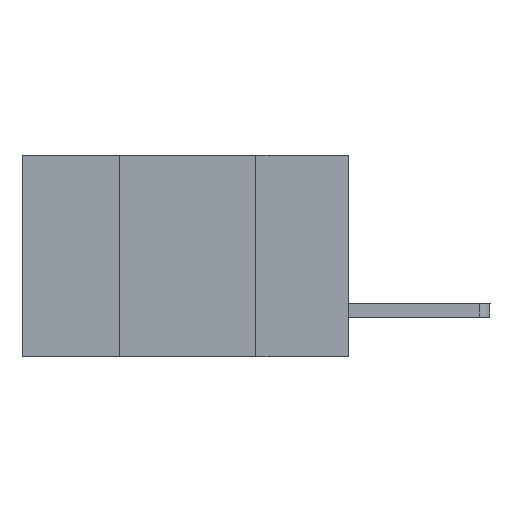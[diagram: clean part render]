
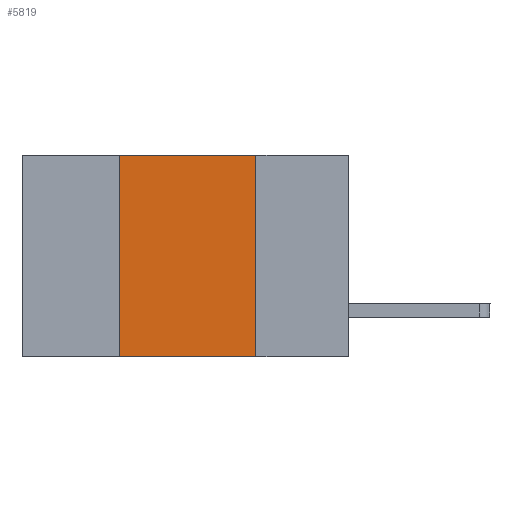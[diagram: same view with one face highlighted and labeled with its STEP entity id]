
A CAD part, left-side view. The second image highlights one B-rep face of the part: STEP entity #5819.
In plain terms, the highlighted planar face has unit normal (-1, 0, 0).
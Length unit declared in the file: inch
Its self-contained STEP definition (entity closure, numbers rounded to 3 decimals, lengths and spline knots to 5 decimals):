
#98 = VECTOR ( 'NONE', #1714, 39.37008 ) ;
#249 = DIRECTION ( 'NONE',  ( 0., -1., 0. ) ) ;
#427 = VECTOR ( 'NONE', #249, 39.37008 ) ;
#1068 = CARTESIAN_POINT ( 'NONE',  ( 0., 0.42, 0. ) ) ;
#1378 = DIRECTION ( 'NONE',  ( 1., 0., 0. ) ) ;
#1493 = VERTEX_POINT ( 'NONE', #8053 ) ;
#1714 = DIRECTION ( 'NONE',  ( 0., 0., 1. ) ) ;
#2317 = EDGE_CURVE ( 'NONE', #6563, #5728, #7318, .T. ) ;
#2407 = CARTESIAN_POINT ( 'NONE',  ( 0., 0.6, 0. ) ) ;
#2536 = LINE ( 'NONE', #5378, #6624 ) ;
#2976 = VERTEX_POINT ( 'NONE', #6179 ) ;
#2998 = ORIENTED_EDGE ( 'NONE', *, *, #7385, .F. ) ;
#3317 = VECTOR ( 'NONE', #5239, 39.37008 ) ;
#3414 = CARTESIAN_POINT ( 'NONE',  ( 0., 0.6, 0. ) ) ;
#4210 = PLANE ( 'NONE',  #8744 ) ;
#4684 = DIRECTION ( 'NONE',  ( 0., 0., -1. ) ) ;
#4859 = EDGE_LOOP ( 'NONE', ( #6746, #2998, #8231, #6671 ) ) ;
#5219 = CARTESIAN_POINT ( 'NONE',  ( 0., 0.42, -0.37 ) ) ;
#5239 = DIRECTION ( 'NONE',  ( 0., -1., 0. ) ) ;
#5378 = CARTESIAN_POINT ( 'NONE',  ( 0., 0.17, 0. ) ) ;
#5475 = DIRECTION ( 'NONE',  ( 0., 0., -1. ) ) ;
#5728 = VERTEX_POINT ( 'NONE', #6873 ) ;
#5819 = ADVANCED_FACE ( 'NONE', ( #6225 ), #4210, .F. ) ;
#5954 = LINE ( 'NONE', #2407, #3317 ) ;
#6179 = CARTESIAN_POINT ( 'NONE',  ( 0., 0.42, 0. ) ) ;
#6225 = FACE_OUTER_BOUND ( 'NONE', #4859, .T. ) ;
#6563 = VERTEX_POINT ( 'NONE', #5219 ) ;
#6624 = VECTOR ( 'NONE', #4684, 39.37008 ) ;
#6671 = ORIENTED_EDGE ( 'NONE', *, *, #2317, .T. ) ;
#6746 = ORIENTED_EDGE ( 'NONE', *, *, #8791, .F. ) ;
#6789 = LINE ( 'NONE', #1068, #98 ) ;
#6873 = CARTESIAN_POINT ( 'NONE',  ( 0., 0.17, -0.37 ) ) ;
#7318 = LINE ( 'NONE', #7497, #427 ) ;
#7385 = EDGE_CURVE ( 'NONE', #2976, #1493, #5954, .T. ) ;
#7497 = CARTESIAN_POINT ( 'NONE',  ( 0., 0.6, -0.37 ) ) ;
#8053 = CARTESIAN_POINT ( 'NONE',  ( 0., 0.17, 0. ) ) ;
#8231 = ORIENTED_EDGE ( 'NONE', *, *, #9140, .F. ) ;
#8744 = AXIS2_PLACEMENT_3D ( 'NONE', #3414, #1378, #5475 ) ;
#8791 = EDGE_CURVE ( 'NONE', #1493, #5728, #2536, .T. ) ;
#9140 = EDGE_CURVE ( 'NONE', #6563, #2976, #6789, .T. ) ;
